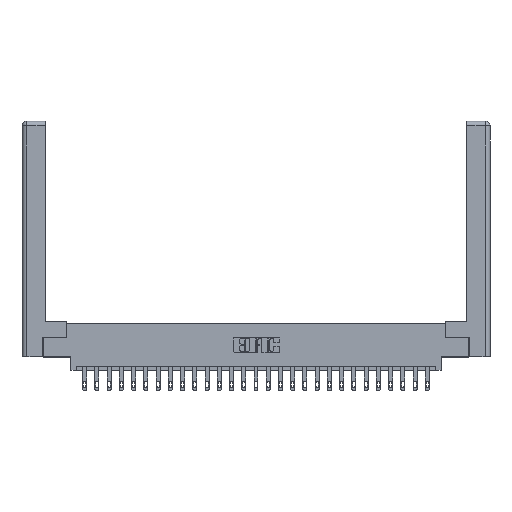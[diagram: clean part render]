
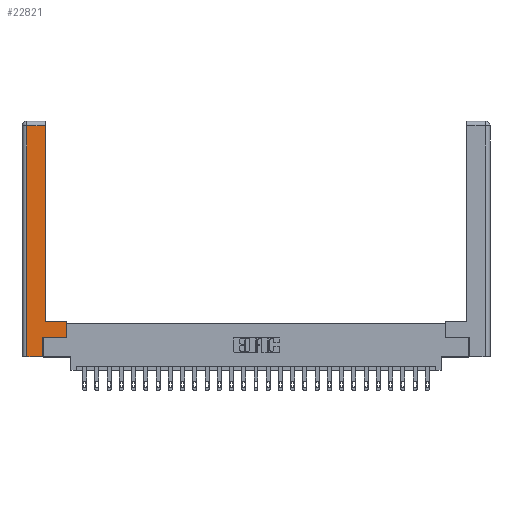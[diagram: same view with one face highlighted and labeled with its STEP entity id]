
A CAD part, top view. The second image highlights one B-rep face of the part: STEP entity #22821.
In plain terms, the highlighted planar face has unit normal (0, 0, 1).
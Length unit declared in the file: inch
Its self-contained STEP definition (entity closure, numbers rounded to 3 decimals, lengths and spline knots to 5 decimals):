
#22 = AXIS2_PLACEMENT_3D ( 'NONE', #5123, #6933, #7115 ) ;
#154 = DIRECTION ( 'NONE',  ( 0., -1., 0. ) ) ;
#340 = LINE ( 'NONE', #10464, #15934 ) ;
#760 = VERTEX_POINT ( 'NONE', #23973 ) ;
#774 = DIRECTION ( 'NONE',  ( 0., 1., 0. ) ) ;
#1197 = VERTEX_POINT ( 'NONE', #22688 ) ;
#1431 = VERTEX_POINT ( 'NONE', #14080 ) ;
#1481 = VERTEX_POINT ( 'NONE', #4055 ) ;
#1670 = EDGE_CURVE ( 'NONE', #8649, #17672, #8673, .T. ) ;
#2289 = CARTESIAN_POINT ( 'NONE',  ( 0.0615, 2.94, 0. ) ) ;
#3124 = DIRECTION ( 'NONE',  ( 0., 1., 0. ) ) ;
#3435 = FACE_OUTER_BOUND ( 'NONE', #16754, .T. ) ;
#3609 = ORIENTED_EDGE ( 'NONE', *, *, #8031, .T. ) ;
#4055 = CARTESIAN_POINT ( 'NONE',  ( 0.265, 0., 0. ) ) ;
#5070 = VERTEX_POINT ( 'NONE', #8779 ) ;
#5085 = VECTOR ( 'NONE', #20677, 39.37008 ) ;
#5123 = CARTESIAN_POINT ( 'NONE',  ( 0., 0., 0. ) ) ;
#6049 = LINE ( 'NONE', #16899, #23344 ) ;
#6106 = CARTESIAN_POINT ( 'NONE',  ( 0.0615, 2.94, 0. ) ) ;
#6178 = ORIENTED_EDGE ( 'NONE', *, *, #20652, .T. ) ;
#6266 = LINE ( 'NONE', #17215, #16078 ) ;
#6516 = CARTESIAN_POINT ( 'NONE',  ( 0.295, 3., 0. ) ) ;
#6578 = EDGE_CURVE ( 'NONE', #1481, #1431, #15906, .T. ) ;
#6933 = DIRECTION ( 'NONE',  ( 0., 0., -1. ) ) ;
#7115 = DIRECTION ( 'NONE',  ( -1., 0., 0. ) ) ;
#8031 = EDGE_CURVE ( 'NONE', #17672, #5070, #340, .T. ) ;
#8170 = EDGE_CURVE ( 'NONE', #5070, #1481, #15265, .T. ) ;
#8649 = VERTEX_POINT ( 'NONE', #17114 ) ;
#8673 = LINE ( 'NONE', #2289, #5085 ) ;
#8727 = LINE ( 'NONE', #6516, #20475 ) ;
#8730 = VECTOR ( 'NONE', #3124, 39.37008 ) ;
#8779 = CARTESIAN_POINT ( 'NONE',  ( 0.0615, 0., 0. ) ) ;
#8988 = CARTESIAN_POINT ( 'NONE',  ( 0.295, 0.45, 0. ) ) ;
#9838 = EDGE_CURVE ( 'NONE', #1431, #760, #6049, .T. ) ;
#10464 = CARTESIAN_POINT ( 'NONE',  ( 0.0615, 0., 0. ) ) ;
#11065 = VECTOR ( 'NONE', #23553, 39.37008 ) ;
#11890 = EDGE_CURVE ( 'NONE', #760, #24333, #6266, .T. ) ;
#12812 = ORIENTED_EDGE ( 'NONE', *, *, #8170, .T. ) ;
#13019 = EDGE_CURVE ( 'NONE', #24333, #1197, #18918, .T. ) ;
#14080 = CARTESIAN_POINT ( 'NONE',  ( 0.265, 0.245, 0. ) ) ;
#15265 = LINE ( 'NONE', #24398, #23075 ) ;
#15906 = LINE ( 'NONE', #26133, #8730 ) ;
#15934 = VECTOR ( 'NONE', #154, 39.37008 ) ;
#16078 = VECTOR ( 'NONE', #774, 39.37008 ) ;
#16754 = EDGE_LOOP ( 'NONE', ( #6178, #20574, #3609, #12812, #18041, #16796, #20986, #25333 ) ) ;
#16796 = ORIENTED_EDGE ( 'NONE', *, *, #9838, .T. ) ;
#16899 = CARTESIAN_POINT ( 'NONE',  ( 0.565, 0.245, 0. ) ) ;
#17114 = CARTESIAN_POINT ( 'NONE',  ( 0.295, 2.94, 0. ) ) ;
#17215 = CARTESIAN_POINT ( 'NONE',  ( 0.565, 0.45, 0. ) ) ;
#17342 = PLANE ( 'NONE',  #22 ) ;
#17672 = VERTEX_POINT ( 'NONE', #6106 ) ;
#18041 = ORIENTED_EDGE ( 'NONE', *, *, #6578, .T. ) ;
#18918 = LINE ( 'NONE', #8988, #11065 ) ;
#20475 = VECTOR ( 'NONE', #22934, 39.37008 ) ;
#20574 = ORIENTED_EDGE ( 'NONE', *, *, #1670, .T. ) ;
#20652 = EDGE_CURVE ( 'NONE', #1197, #8649, #8727, .T. ) ;
#20677 = DIRECTION ( 'NONE',  ( -1., 0., 0. ) ) ;
#20986 = ORIENTED_EDGE ( 'NONE', *, *, #11890, .T. ) ;
#22688 = CARTESIAN_POINT ( 'NONE',  ( 0.295, 0.45, 0. ) ) ;
#22821 = ADVANCED_FACE ( 'NONE', ( #3435 ), #17342, .F. ) ;
#22934 = DIRECTION ( 'NONE',  ( 0., 1., 0. ) ) ;
#23075 = VECTOR ( 'NONE', #26312, 39.37008 ) ;
#23344 = VECTOR ( 'NONE', #25039, 39.37008 ) ;
#23553 = DIRECTION ( 'NONE',  ( -1., 0., 0. ) ) ;
#23973 = CARTESIAN_POINT ( 'NONE',  ( 0.565, 0.245, 0. ) ) ;
#24333 = VERTEX_POINT ( 'NONE', #25118 ) ;
#24398 = CARTESIAN_POINT ( 'NONE',  ( 0.265, 0., 0. ) ) ;
#25039 = DIRECTION ( 'NONE',  ( 1., 0., 0. ) ) ;
#25118 = CARTESIAN_POINT ( 'NONE',  ( 0.565, 0.45, 0. ) ) ;
#25333 = ORIENTED_EDGE ( 'NONE', *, *, #13019, .T. ) ;
#26133 = CARTESIAN_POINT ( 'NONE',  ( 0.265, 0.245, 0. ) ) ;
#26312 = DIRECTION ( 'NONE',  ( 1., 0., 0. ) ) ;
